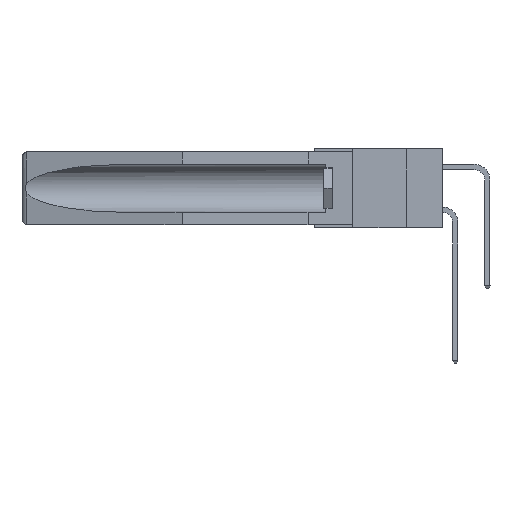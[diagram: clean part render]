
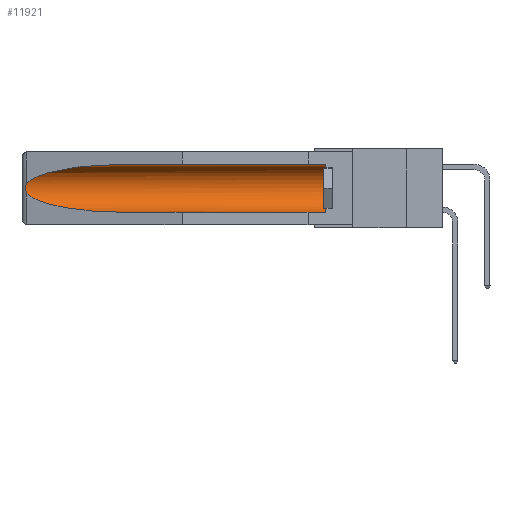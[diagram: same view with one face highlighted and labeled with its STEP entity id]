
A CAD part, left-side view. The second image highlights one B-rep face of the part: STEP entity #11921.
In plain terms, the highlighted cylindrical face has radius 2.857 mm (diameter 5.715 mm), a partial arc.
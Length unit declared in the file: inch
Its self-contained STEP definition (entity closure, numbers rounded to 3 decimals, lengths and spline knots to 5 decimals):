
#50 = CARTESIAN_POINT ( 'NONE',  ( 0.26537, 1.52718, -0.14972 ) ) ;
#218 = CARTESIAN_POINT ( 'NONE',  ( 0.2673, 1.53269, -0.17917 ) ) ;
#687 = LINE ( 'NONE', #9638, #8903 ) ;
#760 = DIRECTION ( 'NONE',  ( 0., 1., 0. ) ) ;
#1428 = CARTESIAN_POINT ( 'NONE',  ( 0.2675, 1.53308, -0.17534 ) ) ;
#1474 = DIRECTION ( 'NONE',  ( 0., 0., 1. ) ) ;
#1488 = CARTESIAN_POINT ( 'NONE',  ( 0.26537, 1.52718, -0.14972 ) ) ;
#1601 = CARTESIAN_POINT ( 'NONE',  ( 0.26537, 1.52718, -0.19328 ) ) ;
#1692 = EDGE_CURVE ( 'NONE', #2893, #6170, #17298, .T. ) ;
#1744 = CARTESIAN_POINT ( 'NONE',  ( 0.155, 1.07973, -0.284 ) ) ;
#2550 =( BOUNDED_CURVE ( )  B_SPLINE_CURVE ( 3, ( #13323, #17785, #9826, #11343 ),
 .UNSPECIFIED., .F., .F. ) 
 B_SPLINE_CURVE_WITH_KNOTS ( ( 4, 4 ),
 ( 0.1948, 1.5708 ),
 .UNSPECIFIED. ) 
 CURVE ( )  GEOMETRIC_REPRESENTATION_ITEM ( )  RATIONAL_B_SPLINE_CURVE ( ( 1., 0.848, 0.848, 1. ) ) 
 REPRESENTATION_ITEM ( '' )  );
#2893 = VERTEX_POINT ( 'NONE', #3382 ) ;
#3009 = AXIS2_PLACEMENT_3D ( 'NONE', #9209, #760, #16311 ) ;
#3382 = CARTESIAN_POINT ( 'NONE',  ( 0.155, 1.07973, -0.059 ) ) ;
#3455 = CARTESIAN_POINT ( 'NONE',  ( 0.155, 0.126, -0.284 ) ) ;
#3635 = CARTESIAN_POINT ( 'NONE',  ( 0.155, 0.126, -0.059 ) ) ;
#5327 = ORIENTED_EDGE ( 'NONE', *, *, #1692, .T. ) ;
#5441 = DIRECTION ( 'NONE',  ( 0., 1., 0. ) ) ;
#5564 = CARTESIAN_POINT ( 'NONE',  ( 0.155, 1.07973, -0.059 ) ) ;
#5613 = ORIENTED_EDGE ( 'NONE', *, *, #15024, .T. ) ;
#5644 = VERTEX_POINT ( 'NONE', #1744 ) ;
#5810 = AXIS2_PLACEMENT_3D ( 'NONE', #7206, #7326, #1474 ) ;
#5984 = CARTESIAN_POINT ( 'NONE',  ( 0.26537, 1.52718, -0.19328 ) ) ;
#5989 = CARTESIAN_POINT ( 'NONE',  ( 0.26654, 1.53092, -0.15636 ) ) ;
#6044 = VERTEX_POINT ( 'NONE', #5984 ) ;
#6170 = VERTEX_POINT ( 'NONE', #14909 ) ;
#6442 = ORIENTED_EDGE ( 'NONE', *, *, #16274, .T. ) ;
#6486 = CYLINDRICAL_SURFACE ( 'NONE', #3009, 0.1125 ) ;
#6765 = DIRECTION ( 'NONE',  ( 0., 1., 0. ) ) ;
#7206 = CARTESIAN_POINT ( 'NONE',  ( 0.155, 0.126, -0.1715 ) ) ;
#7219 = CARTESIAN_POINT ( 'NONE',  ( 0.2675, 1.53308, -0.16763 ) ) ;
#7226 = CARTESIAN_POINT ( 'NONE',  ( 0.21114, 1.30732, -0.059 ) ) ;
#7326 = DIRECTION ( 'NONE',  ( 0., -1., 0. ) ) ;
#7726 = VERTEX_POINT ( 'NONE', #3635 ) ;
#7972 = VERTEX_POINT ( 'NONE', #3455 ) ;
#8396 = CARTESIAN_POINT ( 'NONE',  ( 0.25451, 1.48313, -0.09465 ) ) ;
#8702 = CARTESIAN_POINT ( 'NONE',  ( 0.26597, 1.52961, -0.15275 ) ) ;
#8903 = VECTOR ( 'NONE', #5441, 39.37008 ) ;
#9209 = CARTESIAN_POINT ( 'NONE',  ( 0.155, -0.30754, -0.1715 ) ) ;
#9638 = CARTESIAN_POINT ( 'NONE',  ( 0.155, -0.30754, -0.284 ) ) ;
#9826 = CARTESIAN_POINT ( 'NONE',  ( 0.21114, 1.30732, -0.284 ) ) ;
#9854 = CIRCLE ( 'NONE', #5810, 0.1125 ) ;
#10096 = CARTESIAN_POINT ( 'NONE',  ( 0.26655, 1.53094, -0.18657 ) ) ;
#10720 = VECTOR ( 'NONE', #6765, 39.37008 ) ;
#10934 = ORIENTED_EDGE ( 'NONE', *, *, #15783, .T. ) ;
#10936 = ORIENTED_EDGE ( 'NONE', *, *, #12295, .F. ) ;
#11343 = CARTESIAN_POINT ( 'NONE',  ( 0.155, 1.07973, -0.284 ) ) ;
#11375 = CARTESIAN_POINT ( 'NONE',  ( 0.26597, 1.5296, -0.19026 ) ) ;
#11921 = ADVANCED_FACE ( 'NONE', ( #13079 ), #6486, .F. ) ;
#12295 = EDGE_CURVE ( 'NONE', #7972, #5644, #687, .T. ) ;
#13079 = FACE_OUTER_BOUND ( 'NONE', #13429, .T. ) ;
#13323 = CARTESIAN_POINT ( 'NONE',  ( 0.26537, 1.52718, -0.19328 ) ) ;
#13429 = EDGE_LOOP ( 'NONE', ( #5327, #10934, #5613, #10936, #18191, #6442 ) ) ;
#14276 = B_SPLINE_CURVE_WITH_KNOTS ( 'NONE', 3,
 ( #1488, #8702, #5989, #16952, #7219, #1428, #218, #10096, #11375, #1601 ),
 .UNSPECIFIED., .F., .F.,
 ( 4, 2, 2, 2, 4 ),
 ( 0., 0.00029, 0.00058, 0.00087, 0.00117 ),
 .UNSPECIFIED. ) ;
#14909 = CARTESIAN_POINT ( 'NONE',  ( 0.26537, 1.52718, -0.14972 ) ) ;
#15024 = EDGE_CURVE ( 'NONE', #6044, #5644, #2550, .T. ) ;
#15229 = CARTESIAN_POINT ( 'NONE',  ( 0.155, -0.30754, -0.059 ) ) ;
#15783 = EDGE_CURVE ( 'NONE', #6170, #6044, #14276, .T. ) ;
#16274 = EDGE_CURVE ( 'NONE', #7726, #2893, #17737, .T. ) ;
#16311 = DIRECTION ( 'NONE',  ( 0., 0., 1. ) ) ;
#16536 = EDGE_CURVE ( 'NONE', #7972, #7726, #9854, .T. ) ;
#16952 = CARTESIAN_POINT ( 'NONE',  ( 0.2673, 1.5327, -0.16383 ) ) ;
#17298 =( BOUNDED_CURVE ( )  B_SPLINE_CURVE ( 3, ( #5564, #7226, #8396, #50 ),
 .UNSPECIFIED., .F., .T. ) 
 B_SPLINE_CURVE_WITH_KNOTS ( ( 4, 4 ),
 ( 4.71239, 6.08839 ),
 .UNSPECIFIED. ) 
 CURVE ( )  GEOMETRIC_REPRESENTATION_ITEM ( )  RATIONAL_B_SPLINE_CURVE ( ( 1., 0.848, 0.848, 1. ) ) 
 REPRESENTATION_ITEM ( '' )  );
#17737 = LINE ( 'NONE', #15229, #10720 ) ;
#17785 = CARTESIAN_POINT ( 'NONE',  ( 0.25451, 1.48313, -0.24835 ) ) ;
#18191 = ORIENTED_EDGE ( 'NONE', *, *, #16536, .T. ) ;
